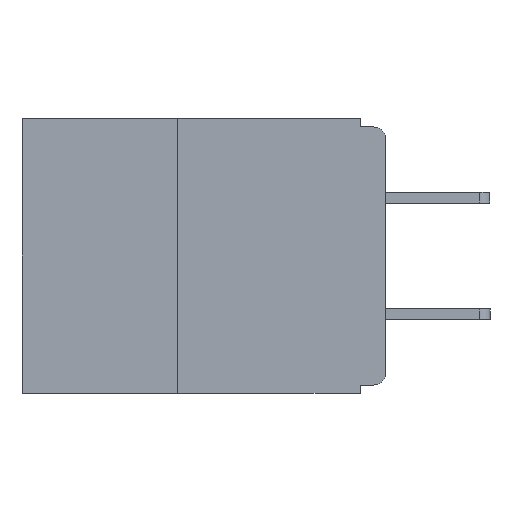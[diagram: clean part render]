
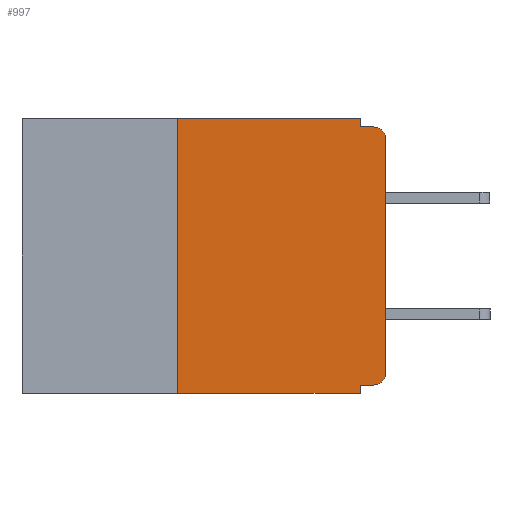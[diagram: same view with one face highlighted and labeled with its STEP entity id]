
A CAD part, left-side view. The second image highlights one B-rep face of the part: STEP entity #997.
In plain terms, the highlighted planar face has unit normal (-1, 0, 0).
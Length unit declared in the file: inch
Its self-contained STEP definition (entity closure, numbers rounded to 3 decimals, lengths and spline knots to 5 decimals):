
#824 = DIRECTION ( 'NONE',  ( 1., 0., 0. ) ) ;
#997 = ADVANCED_FACE ( 'NONE', ( #7207 ), #3382, .F. ) ;
#1173 = EDGE_LOOP ( 'NONE', ( #15217, #5746, #11037, #21879, #23535, #24516, #16531, #18873, #21998, #30540 ) ) ;
#1367 = DIRECTION ( 'NONE',  ( 0., 0., -1. ) ) ;
#3173 = DIRECTION ( 'NONE',  ( 0., -1., 0. ) ) ;
#3382 = PLANE ( 'NONE',  #22037 ) ;
#4099 = CARTESIAN_POINT ( 'NONE',  ( 0., 0.25, -0.33 ) ) ;
#4547 = CARTESIAN_POINT ( 'NONE',  ( 0., 0.031, -0.33 ) ) ;
#4889 = LINE ( 'NONE', #11022, #24519 ) ;
#5057 = LINE ( 'NONE', #30162, #23911 ) ;
#5226 = EDGE_CURVE ( 'NONE', #17081, #25622, #19752, .T. ) ;
#5332 = VECTOR ( 'NONE', #32071, 39.37008 ) ;
#5746 = ORIENTED_EDGE ( 'NONE', *, *, #14908, .T. ) ;
#5988 = VECTOR ( 'NONE', #6053, 39.37008 ) ;
#6009 = CARTESIAN_POINT ( 'NONE',  ( 0., 0.031, -0.33 ) ) ;
#6053 = DIRECTION ( 'NONE',  ( 0., -1., 0. ) ) ;
#6185 = CARTESIAN_POINT ( 'NONE',  ( 0., 0.437, -0.33 ) ) ;
#6995 = VECTOR ( 'NONE', #21844, 39.37008 ) ;
#7207 = FACE_OUTER_BOUND ( 'NONE', #1173, .T. ) ;
#7265 = VECTOR ( 'NONE', #30010, 39.37008 ) ;
#8113 = LINE ( 'NONE', #17588, #7265 ) ;
#8632 = DIRECTION ( 'NONE',  ( 0., 0., -1. ) ) ;
#8746 = VECTOR ( 'NONE', #8632, 39.37008 ) ;
#8976 = CARTESIAN_POINT ( 'NONE',  ( 0., 0.015, -0.305 ) ) ;
#9491 = VERTEX_POINT ( 'NONE', #32464 ) ;
#10576 = VERTEX_POINT ( 'NONE', #31475 ) ;
#10680 = CARTESIAN_POINT ( 'NONE',  ( 0., 0.031, -0.01 ) ) ;
#10807 = EDGE_CURVE ( 'NONE', #14143, #28677, #8113, .T. ) ;
#11022 = CARTESIAN_POINT ( 'NONE',  ( 0., 0., -0.01 ) ) ;
#11037 = ORIENTED_EDGE ( 'NONE', *, *, #25925, .F. ) ;
#11151 = EDGE_CURVE ( 'NONE', #9491, #25622, #29753, .T. ) ;
#11506 = EDGE_CURVE ( 'NONE', #17081, #22891, #5057, .T. ) ;
#11610 = DIRECTION ( 'NONE',  ( 0., 0., -1. ) ) ;
#12525 = CARTESIAN_POINT ( 'NONE',  ( 0., 0.031, 0. ) ) ;
#13299 = DIRECTION ( 'NONE',  ( -1., 0., 0. ) ) ;
#13961 = LINE ( 'NONE', #19329, #6995 ) ;
#14143 = VERTEX_POINT ( 'NONE', #12525 ) ;
#14299 = EDGE_CURVE ( 'NONE', #15340, #9491, #15934, .T. ) ;
#14908 = EDGE_CURVE ( 'NONE', #26274, #31411, #30301, .T. ) ;
#15217 = ORIENTED_EDGE ( 'NONE', *, *, #31546, .T. ) ;
#15340 = VERTEX_POINT ( 'NONE', #24598 ) ;
#15686 = DIRECTION ( 'NONE',  ( 0., 1., 0. ) ) ;
#15934 = LINE ( 'NONE', #28169, #28443 ) ;
#16531 = ORIENTED_EDGE ( 'NONE', *, *, #5226, .T. ) ;
#17081 = VERTEX_POINT ( 'NONE', #4099 ) ;
#17588 = CARTESIAN_POINT ( 'NONE',  ( 0., 0.031, 0. ) ) ;
#17654 = DIRECTION ( 'NONE',  ( 0., 0., 1. ) ) ;
#17974 = EDGE_CURVE ( 'NONE', #15340, #10576, #31421, .T. ) ;
#18873 = ORIENTED_EDGE ( 'NONE', *, *, #11151, .F. ) ;
#19329 = CARTESIAN_POINT ( 'NONE',  ( 0., 0.437, 0. ) ) ;
#19752 = LINE ( 'NONE', #6185, #5988 ) ;
#21258 = AXIS2_PLACEMENT_3D ( 'NONE', #8976, #26796, #11610 ) ;
#21679 = CARTESIAN_POINT ( 'NONE',  ( 0., 0.015, -0.01 ) ) ;
#21844 = DIRECTION ( 'NONE',  ( 0., -1., 0. ) ) ;
#21879 = ORIENTED_EDGE ( 'NONE', *, *, #10807, .F. ) ;
#21998 = ORIENTED_EDGE ( 'NONE', *, *, #14299, .F. ) ;
#22037 = AXIS2_PLACEMENT_3D ( 'NONE', #32110, #824, #1367 ) ;
#22891 = VERTEX_POINT ( 'NONE', #28342 ) ;
#23182 = CARTESIAN_POINT ( 'NONE',  ( 0., 0., -0.025 ) ) ;
#23535 = ORIENTED_EDGE ( 'NONE', *, *, #24766, .F. ) ;
#23911 = VECTOR ( 'NONE', #17654, 39.37008 ) ;
#24516 = ORIENTED_EDGE ( 'NONE', *, *, #11506, .F. ) ;
#24519 = VECTOR ( 'NONE', #3173, 39.37008 ) ;
#24598 = CARTESIAN_POINT ( 'NONE',  ( 0., 0.015, -0.32 ) ) ;
#24766 = EDGE_CURVE ( 'NONE', #22891, #14143, #13961, .T. ) ;
#25622 = VERTEX_POINT ( 'NONE', #4547 ) ;
#25738 = LINE ( 'NONE', #29672, #5332 ) ;
#25925 = EDGE_CURVE ( 'NONE', #28677, #31411, #4889, .T. ) ;
#26274 = VERTEX_POINT ( 'NONE', #23182 ) ;
#26796 = DIRECTION ( 'NONE',  ( -1., 0., 0. ) ) ;
#28169 = CARTESIAN_POINT ( 'NONE',  ( 0., 0., -0.32 ) ) ;
#28342 = CARTESIAN_POINT ( 'NONE',  ( 0., 0.25, 0. ) ) ;
#28354 = CARTESIAN_POINT ( 'NONE',  ( 0., 0.015, -0.025 ) ) ;
#28443 = VECTOR ( 'NONE', #15686, 39.37008 ) ;
#28677 = VERTEX_POINT ( 'NONE', #10680 ) ;
#29308 = AXIS2_PLACEMENT_3D ( 'NONE', #28354, #13299, #30782 ) ;
#29672 = CARTESIAN_POINT ( 'NONE',  ( 0., 0., 0. ) ) ;
#29753 = LINE ( 'NONE', #6009, #8746 ) ;
#30010 = DIRECTION ( 'NONE',  ( 0., 0., -1. ) ) ;
#30162 = CARTESIAN_POINT ( 'NONE',  ( 0., 0.25, -0.33 ) ) ;
#30301 = CIRCLE ( 'NONE', #29308, 0.015 ) ;
#30540 = ORIENTED_EDGE ( 'NONE', *, *, #17974, .T. ) ;
#30782 = DIRECTION ( 'NONE',  ( 0., 0., -1. ) ) ;
#31411 = VERTEX_POINT ( 'NONE', #21679 ) ;
#31421 = CIRCLE ( 'NONE', #21258, 0.015 ) ;
#31475 = CARTESIAN_POINT ( 'NONE',  ( 0., 0., -0.305 ) ) ;
#31546 = EDGE_CURVE ( 'NONE', #10576, #26274, #25738, .T. ) ;
#32071 = DIRECTION ( 'NONE',  ( 0., 0., 1. ) ) ;
#32110 = CARTESIAN_POINT ( 'NONE',  ( 0., 0.437, 0. ) ) ;
#32464 = CARTESIAN_POINT ( 'NONE',  ( 0., 0.031, -0.32 ) ) ;
